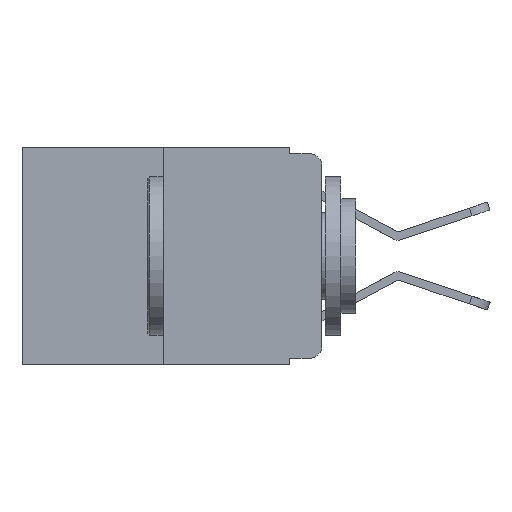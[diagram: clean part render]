
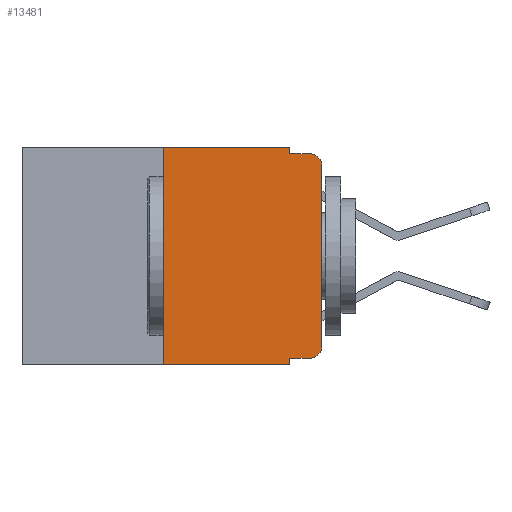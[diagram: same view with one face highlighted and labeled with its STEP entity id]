
A CAD part, left-side view. The second image highlights one B-rep face of the part: STEP entity #13481.
In plain terms, the highlighted planar face has unit normal (-1, 0, 0).
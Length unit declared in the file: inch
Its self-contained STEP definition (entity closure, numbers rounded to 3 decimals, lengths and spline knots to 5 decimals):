
#167 = CARTESIAN_POINT ( 'NONE',  ( 0., 0.473, 0. ) ) ;
#182 = DIRECTION ( 'NONE',  ( 0., -1., 0. ) ) ;
#375 = VECTOR ( 'NONE', #11002, 39.37008 ) ;
#554 = CARTESIAN_POINT ( 'NONE',  ( 0., 0.25, 0. ) ) ;
#669 = CARTESIAN_POINT ( 'NONE',  ( 0., 0.051, 0. ) ) ;
#830 = CARTESIAN_POINT ( 'NONE',  ( 0., 0.473, -0.343 ) ) ;
#928 = ORIENTED_EDGE ( 'NONE', *, *, #8221, .F. ) ;
#931 = DIRECTION ( 'NONE',  ( 0., -1., 0. ) ) ;
#1085 = EDGE_CURVE ( 'NONE', #10008, #6008, #2663, .T. ) ;
#1160 = DIRECTION ( 'NONE',  ( 0., 0., -1. ) ) ;
#1167 = VERTEX_POINT ( 'NONE', #1603 ) ;
#1288 = VERTEX_POINT ( 'NONE', #5068 ) ;
#1578 = ORIENTED_EDGE ( 'NONE', *, *, #7288, .F. ) ;
#1603 = CARTESIAN_POINT ( 'NONE',  ( 0., 0.051, -0.343 ) ) ;
#1862 = DIRECTION ( 'NONE',  ( 0., 0., 1. ) ) ;
#1865 = EDGE_CURVE ( 'NONE', #1288, #1167, #11339, .T. ) ;
#2039 = CARTESIAN_POINT ( 'NONE',  ( 0., 0.051, -0.01 ) ) ;
#2184 = VERTEX_POINT ( 'NONE', #2628 ) ;
#2628 = CARTESIAN_POINT ( 'NONE',  ( 0., 0.02, -0.01 ) ) ;
#2663 = CIRCLE ( 'NONE', #10381, 0.02 ) ;
#2816 = VERTEX_POINT ( 'NONE', #5384 ) ;
#2896 = CIRCLE ( 'NONE', #6222, 0.02 ) ;
#3131 = VECTOR ( 'NONE', #931, 39.37008 ) ;
#3550 = CARTESIAN_POINT ( 'NONE',  ( 0., 0.02, -0.313 ) ) ;
#3636 = DIRECTION ( 'NONE',  ( 1., 0., 0. ) ) ;
#3802 = VECTOR ( 'NONE', #11211, 39.37008 ) ;
#3860 = CARTESIAN_POINT ( 'NONE',  ( 0., 0.051, -0.01 ) ) ;
#4012 = ORIENTED_EDGE ( 'NONE', *, *, #1865, .T. ) ;
#4247 = CARTESIAN_POINT ( 'NONE',  ( 0., 0.02, -0.333 ) ) ;
#4758 = DIRECTION ( 'NONE',  ( 0., 0., -1. ) ) ;
#5068 = CARTESIAN_POINT ( 'NONE',  ( 0., 0.25, -0.343 ) ) ;
#5224 = DIRECTION ( 'NONE',  ( 0., -1., 0. ) ) ;
#5384 = CARTESIAN_POINT ( 'NONE',  ( 0., 0., -0.03 ) ) ;
#5465 = FACE_OUTER_BOUND ( 'NONE', #13241, .T. ) ;
#5831 = CARTESIAN_POINT ( 'NONE',  ( 0., 0.051, -0.333 ) ) ;
#5953 = DIRECTION ( 'NONE',  ( -1., 0., 0. ) ) ;
#6008 = VERTEX_POINT ( 'NONE', #10369 ) ;
#6222 = AXIS2_PLACEMENT_3D ( 'NONE', #8115, #5953, #11465 ) ;
#6338 = ORIENTED_EDGE ( 'NONE', *, *, #12263, .F. ) ;
#6582 = ORIENTED_EDGE ( 'NONE', *, *, #1085, .T. ) ;
#6745 = DIRECTION ( 'NONE',  ( 0., 0., -1. ) ) ;
#6942 = AXIS2_PLACEMENT_3D ( 'NONE', #167, #3636, #12982 ) ;
#7112 = VECTOR ( 'NONE', #5224, 39.37008 ) ;
#7282 = VERTEX_POINT ( 'NONE', #12335 ) ;
#7288 = EDGE_CURVE ( 'NONE', #1288, #8411, #7863, .T. ) ;
#7321 = LINE ( 'NONE', #2039, #3131 ) ;
#7384 = VECTOR ( 'NONE', #1160, 39.37008 ) ;
#7724 = ORIENTED_EDGE ( 'NONE', *, *, #7731, .T. ) ;
#7731 = EDGE_CURVE ( 'NONE', #6008, #2816, #8861, .T. ) ;
#7863 = LINE ( 'NONE', #554, #375 ) ;
#7984 = VECTOR ( 'NONE', #1862, 39.37008 ) ;
#8115 = CARTESIAN_POINT ( 'NONE',  ( 0., 0.02, -0.03 ) ) ;
#8221 = EDGE_CURVE ( 'NONE', #11888, #2184, #7321, .T. ) ;
#8259 = VECTOR ( 'NONE', #4758, 39.37008 ) ;
#8411 = VERTEX_POINT ( 'NONE', #9782 ) ;
#8594 = LINE ( 'NONE', #9670, #12668 ) ;
#8678 = ORIENTED_EDGE ( 'NONE', *, *, #10987, .T. ) ;
#8720 = CARTESIAN_POINT ( 'NONE',  ( 0., 0.051, 0. ) ) ;
#8825 = LINE ( 'NONE', #13039, #8259 ) ;
#8859 = ORIENTED_EDGE ( 'NONE', *, *, #13041, .F. ) ;
#8861 = LINE ( 'NONE', #11965, #7984 ) ;
#9520 = ORIENTED_EDGE ( 'NONE', *, *, #10164, .T. ) ;
#9654 = PLANE ( 'NONE',  #6942 ) ;
#9670 = CARTESIAN_POINT ( 'NONE',  ( 0., 0.473, 0. ) ) ;
#9782 = CARTESIAN_POINT ( 'NONE',  ( 0., 0.25, 0. ) ) ;
#10008 = VERTEX_POINT ( 'NONE', #4247 ) ;
#10050 = ORIENTED_EDGE ( 'NONE', *, *, #12978, .F. ) ;
#10164 = EDGE_CURVE ( 'NONE', #2816, #2184, #2896, .T. ) ;
#10369 = CARTESIAN_POINT ( 'NONE',  ( 0., 0., -0.313 ) ) ;
#10381 = AXIS2_PLACEMENT_3D ( 'NONE', #3550, #11978, #6745 ) ;
#10987 = EDGE_CURVE ( 'NONE', #7282, #10008, #11137, .T. ) ;
#11002 = DIRECTION ( 'NONE',  ( 0., 0., 1. ) ) ;
#11137 = LINE ( 'NONE', #5831, #3802 ) ;
#11211 = DIRECTION ( 'NONE',  ( 0., -1., 0. ) ) ;
#11339 = LINE ( 'NONE', #830, #7112 ) ;
#11465 = DIRECTION ( 'NONE',  ( 0., 0., -1. ) ) ;
#11602 = LINE ( 'NONE', #8720, #7384 ) ;
#11888 = VERTEX_POINT ( 'NONE', #3860 ) ;
#11965 = CARTESIAN_POINT ( 'NONE',  ( 0., 0., 0. ) ) ;
#11978 = DIRECTION ( 'NONE',  ( -1., 0., 0. ) ) ;
#12263 = EDGE_CURVE ( 'NONE', #7282, #1167, #8825, .T. ) ;
#12335 = CARTESIAN_POINT ( 'NONE',  ( 0., 0.051, -0.333 ) ) ;
#12668 = VECTOR ( 'NONE', #182, 39.37008 ) ;
#12758 = VERTEX_POINT ( 'NONE', #669 ) ;
#12978 = EDGE_CURVE ( 'NONE', #12758, #11888, #11602, .T. ) ;
#12982 = DIRECTION ( 'NONE',  ( 0., 0., -1. ) ) ;
#13039 = CARTESIAN_POINT ( 'NONE',  ( 0., 0.051, 0. ) ) ;
#13041 = EDGE_CURVE ( 'NONE', #8411, #12758, #8594, .T. ) ;
#13241 = EDGE_LOOP ( 'NONE', ( #7724, #9520, #928, #10050, #8859, #1578, #4012, #6338, #8678, #6582 ) ) ;
#13481 = ADVANCED_FACE ( 'NONE', ( #5465 ), #9654, .F. ) ;
